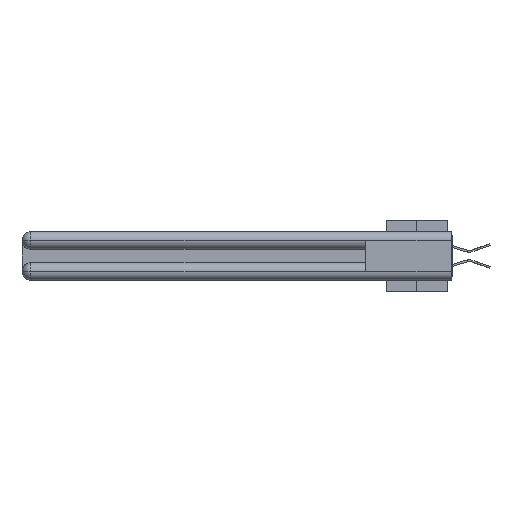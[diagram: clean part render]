
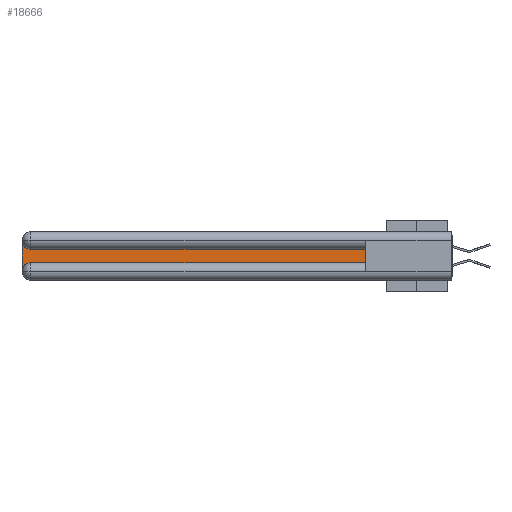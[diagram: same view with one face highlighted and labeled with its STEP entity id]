
A CAD part, left-side view. The second image highlights one B-rep face of the part: STEP entity #18666.
In plain terms, the highlighted planar face has unit normal (-1, 0, 0).
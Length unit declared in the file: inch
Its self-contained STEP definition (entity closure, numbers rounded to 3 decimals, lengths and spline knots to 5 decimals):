
#134 = CARTESIAN_POINT ( 'NONE',  ( 0.075, 3., -0.0625 ) ) ;
#677 = ORIENTED_EDGE ( 'NONE', *, *, #33184, .T. ) ;
#1624 = VERTEX_POINT ( 'NONE', #9296 ) ;
#2193 = LINE ( 'NONE', #11798, #3928 ) ;
#2465 = ORIENTED_EDGE ( 'NONE', *, *, #32022, .T. ) ;
#2689 = DIRECTION ( 'NONE',  ( 0., 0., 1. ) ) ;
#3195 = DIRECTION ( 'NONE',  ( 1., 0., 0. ) ) ;
#3374 = ORIENTED_EDGE ( 'NONE', *, *, #42115, .T. ) ;
#3647 = DIRECTION ( 'NONE',  ( 0., 0., -1. ) ) ;
#3928 = VECTOR ( 'NONE', #48717, 39.37008 ) ;
#4916 = VERTEX_POINT ( 'NONE', #41346 ) ;
#6910 = EDGE_CURVE ( 'NONE', #10007, #14344, #27056, .T. ) ;
#9296 = CARTESIAN_POINT ( 'NONE',  ( 0.075, 2.94, -0.1225 ) ) ;
#10007 = VERTEX_POINT ( 'NONE', #44479 ) ;
#10422 = AXIS2_PLACEMENT_3D ( 'NONE', #12368, #45816, #31341 ) ;
#10721 = DIRECTION ( 'NONE',  ( 0., 0., -1. ) ) ;
#11783 = VECTOR ( 'NONE', #3647, 39.37008 ) ;
#11798 = CARTESIAN_POINT ( 'NONE',  ( 0.075, 0.6, -0.2175 ) ) ;
#11822 = ORIENTED_EDGE ( 'NONE', *, *, #6910, .T. ) ;
#12335 = AXIS2_PLACEMENT_3D ( 'NONE', #30952, #23733, #45565 ) ;
#12368 = CARTESIAN_POINT ( 'NONE',  ( 0.075, 2.94, -0.0625 ) ) ;
#12950 = EDGE_CURVE ( 'NONE', #14344, #20678, #2193, .T. ) ;
#13238 = CARTESIAN_POINT ( 'NONE',  ( 0.075, 0.6, -0.1225 ) ) ;
#14344 = VERTEX_POINT ( 'NONE', #17038 ) ;
#14666 = CARTESIAN_POINT ( 'NONE',  ( 0.075, 3., -0.1225 ) ) ;
#17038 = CARTESIAN_POINT ( 'NONE',  ( 0.075, 2.94, -0.2175 ) ) ;
#17249 = EDGE_LOOP ( 'NONE', ( #2465, #3374, #677, #11822, #19631, #31738 ) ) ;
#18362 = VECTOR ( 'NONE', #2689, 39.37008 ) ;
#18666 = ADVANCED_FACE ( 'NONE', ( #39615 ), #48459, .F. ) ;
#18994 = CARTESIAN_POINT ( 'NONE',  ( 0.075, 0.6, -0.2175 ) ) ;
#19631 = ORIENTED_EDGE ( 'NONE', *, *, #12950, .T. ) ;
#20100 = AXIS2_PLACEMENT_3D ( 'NONE', #14666, #3195, #10721 ) ;
#20678 = VERTEX_POINT ( 'NONE', #18994 ) ;
#20800 = CIRCLE ( 'NONE', #10422, 0.06 ) ;
#22524 = LINE ( 'NONE', #47127, #18362 ) ;
#23733 = DIRECTION ( 'NONE',  ( 1., 0., 0. ) ) ;
#24115 = EDGE_CURVE ( 'NONE', #20678, #4916, #22524, .T. ) ;
#26084 = CARTESIAN_POINT ( 'NONE',  ( 0.075, 3., -0.2175 ) ) ;
#27056 = CIRCLE ( 'NONE', #12335, 0.06 ) ;
#28108 = DIRECTION ( 'NONE',  ( 0., 1., 0. ) ) ;
#30813 = VECTOR ( 'NONE', #28108, 39.37008 ) ;
#30952 = CARTESIAN_POINT ( 'NONE',  ( 0.075, 2.94, -0.2775 ) ) ;
#31341 = DIRECTION ( 'NONE',  ( 0., 0., -1. ) ) ;
#31738 = ORIENTED_EDGE ( 'NONE', *, *, #24115, .T. ) ;
#31860 = LINE ( 'NONE', #26084, #11783 ) ;
#32022 = EDGE_CURVE ( 'NONE', #4916, #1624, #40793, .T. ) ;
#33184 = EDGE_CURVE ( 'NONE', #43664, #10007, #31860, .T. ) ;
#39615 = FACE_OUTER_BOUND ( 'NONE', #17249, .T. ) ;
#40793 = LINE ( 'NONE', #13238, #30813 ) ;
#41346 = CARTESIAN_POINT ( 'NONE',  ( 0.075, 0.6, -0.1225 ) ) ;
#42115 = EDGE_CURVE ( 'NONE', #1624, #43664, #20800, .T. ) ;
#43664 = VERTEX_POINT ( 'NONE', #134 ) ;
#44479 = CARTESIAN_POINT ( 'NONE',  ( 0.075, 3., -0.2775 ) ) ;
#45565 = DIRECTION ( 'NONE',  ( 0., 0., -1. ) ) ;
#45816 = DIRECTION ( 'NONE',  ( 1., 0., 0. ) ) ;
#47127 = CARTESIAN_POINT ( 'NONE',  ( 0.075, 0.6, -0.2175 ) ) ;
#48459 = PLANE ( 'NONE',  #20100 ) ;
#48717 = DIRECTION ( 'NONE',  ( 0., -1., 0. ) ) ;
